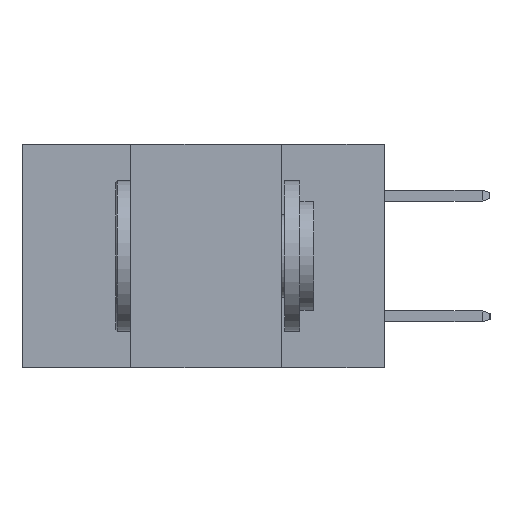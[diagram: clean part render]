
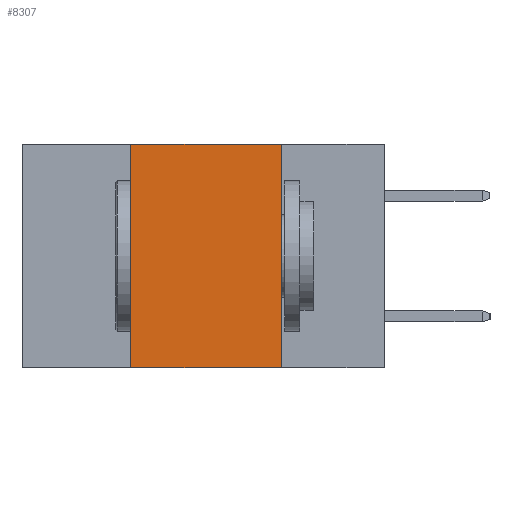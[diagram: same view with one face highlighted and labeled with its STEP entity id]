
A CAD part, left-side view. The second image highlights one B-rep face of the part: STEP entity #8307.
In plain terms, the highlighted planar face has unit normal (-1, 0, 0).
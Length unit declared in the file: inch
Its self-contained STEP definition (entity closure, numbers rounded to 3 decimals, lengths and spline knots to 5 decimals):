
#210 = CARTESIAN_POINT ( 'NONE',  ( 0., 0.6, 0. ) ) ;
#267 = CARTESIAN_POINT ( 'NONE',  ( 0., 0.17, -0.37 ) ) ;
#869 = CARTESIAN_POINT ( 'NONE',  ( 0., 0.42, -0.37 ) ) ;
#1253 = DIRECTION ( 'NONE',  ( 0., 0., -1. ) ) ;
#1305 = DIRECTION ( 'NONE',  ( 0., -1., 0. ) ) ;
#1508 = EDGE_CURVE ( 'NONE', #10240, #11690, #4971, .T. ) ;
#1573 = EDGE_CURVE ( 'NONE', #3478, #10240, #10876, .T. ) ;
#1625 = EDGE_CURVE ( 'NONE', #3478, #3561, #9859, .T. ) ;
#1780 = EDGE_CURVE ( 'NONE', #11690, #3561, #8373, .T. ) ;
#2186 = ORIENTED_EDGE ( 'NONE', *, *, #1625, .T. ) ;
#2381 = VECTOR ( 'NONE', #4530, 39.37008 ) ;
#2469 = AXIS2_PLACEMENT_3D ( 'NONE', #210, #7113, #1253 ) ;
#2527 = ORIENTED_EDGE ( 'NONE', *, *, #1573, .F. ) ;
#2687 = DIRECTION ( 'NONE',  ( 0., 0., 1. ) ) ;
#3452 = CARTESIAN_POINT ( 'NONE',  ( 0., 0.6, -0.37 ) ) ;
#3478 = VERTEX_POINT ( 'NONE', #869 ) ;
#3561 = VERTEX_POINT ( 'NONE', #267 ) ;
#4239 = CARTESIAN_POINT ( 'NONE',  ( 0., 0.42, -0.37 ) ) ;
#4530 = DIRECTION ( 'NONE',  ( 0., -1., 0. ) ) ;
#4971 = LINE ( 'NONE', #7710, #2381 ) ;
#5009 = EDGE_LOOP ( 'NONE', ( #9032, #7842, #2527, #2186 ) ) ;
#5234 = PLANE ( 'NONE',  #2469 ) ;
#5422 = VECTOR ( 'NONE', #1305, 39.37008 ) ;
#6033 = VECTOR ( 'NONE', #2687, 39.37008 ) ;
#6297 = VECTOR ( 'NONE', #10659, 39.37008 ) ;
#6469 = FACE_OUTER_BOUND ( 'NONE', #5009, .T. ) ;
#6760 = CARTESIAN_POINT ( 'NONE',  ( 0., 0.42, 0. ) ) ;
#7113 = DIRECTION ( 'NONE',  ( 1., 0., 0. ) ) ;
#7710 = CARTESIAN_POINT ( 'NONE',  ( 0., 0.6, 0. ) ) ;
#7842 = ORIENTED_EDGE ( 'NONE', *, *, #1508, .F. ) ;
#8307 = ADVANCED_FACE ( 'NONE', ( #6469 ), #5234, .F. ) ;
#8373 = LINE ( 'NONE', #9702, #6297 ) ;
#9032 = ORIENTED_EDGE ( 'NONE', *, *, #1780, .F. ) ;
#9702 = CARTESIAN_POINT ( 'NONE',  ( 0., 0.17, -0.37 ) ) ;
#9859 = LINE ( 'NONE', #3452, #5422 ) ;
#10240 = VERTEX_POINT ( 'NONE', #6760 ) ;
#10659 = DIRECTION ( 'NONE',  ( 0., 0., -1. ) ) ;
#10876 = LINE ( 'NONE', #4239, #6033 ) ;
#11393 = CARTESIAN_POINT ( 'NONE',  ( 0., 0.17, 0. ) ) ;
#11690 = VERTEX_POINT ( 'NONE', #11393 ) ;
